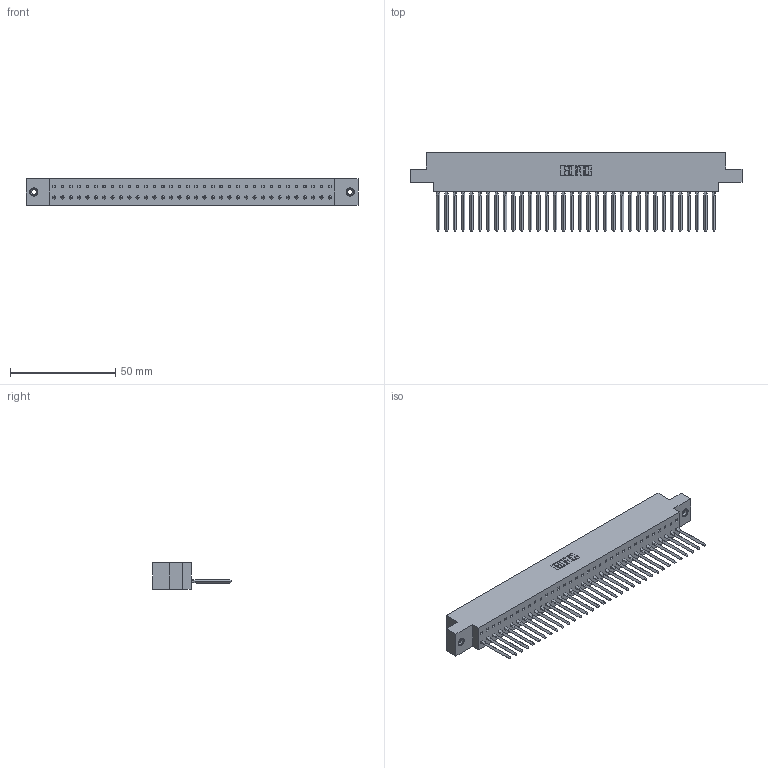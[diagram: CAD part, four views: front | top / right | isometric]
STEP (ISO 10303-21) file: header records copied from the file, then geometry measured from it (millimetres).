
FILE_DESCRIPTION (( 'STEP AP203' ), '1' );
FILE_NAME ('317-034-541-678.STEP', '2020-02-27T21:52:17', ( '' ), ( '' ), 'SwSTEP 2.0', 'SolidWorks 2016', '' );
FILE_SCHEMA (( 'CONFIG_CONTROL_DESIGN' ));
Length unit declared in the file: inch
Products named in the file (4): 317-034-541-678; 345-250-001_345-250-003-102; 317-290-002_541; 317 Part_.156 Dia - TI
Assembly tree (37 placements, depth 2):
  317-034-541-678
    317 Part_.156 Dia - TI
    317-290-002_541  x34
    345-250-001_345-250-003-102  x2
Bounding box: 157.43 x 37.34 x 12.7 mm (x, y, z)
Volume: 25277.2 mm3; surface area: 35473.2 mm2
Topology: 37 solids, 37 shells, 5330 faces, 15167 edges, 9854 vertices
Faces by surface type: plane 4306, cylinder 872, bspline 136, cone 12, torus 4
Entity records: 51909 total; most frequent: CARTESIAN_POINT 9834, ORIENTED_EDGE 9114, DIRECTION 7523, EDGE_CURVE 4557, LINE 4173, VECTOR 4173, VERTEX_POINT 3026, AXIS2_PLACEMENT_3D 1675
